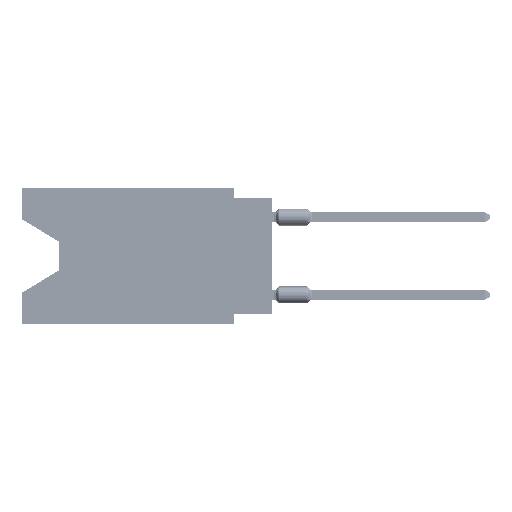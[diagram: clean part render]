
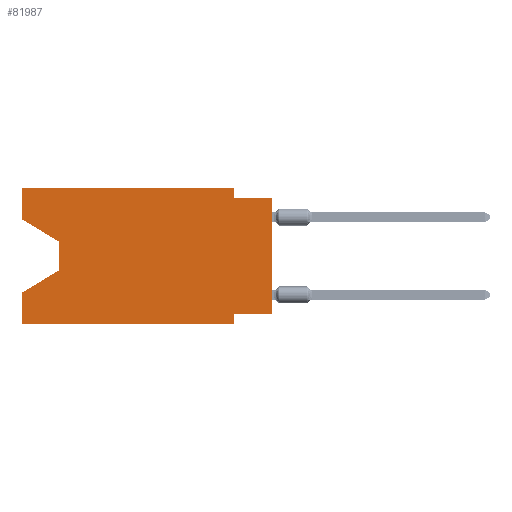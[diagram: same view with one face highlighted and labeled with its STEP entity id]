
A CAD part, left-side view. The second image highlights one B-rep face of the part: STEP entity #81987.
In plain terms, the highlighted planar face has unit normal (-1, 0, 0).
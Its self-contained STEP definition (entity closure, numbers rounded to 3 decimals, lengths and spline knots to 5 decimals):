
#1420 = ORIENTED_EDGE ( 'NONE', *, *, #66123, .F. ) ;
#2248 = CARTESIAN_POINT ( 'NONE',  ( 0., 0.1, 0. ) ) ;
#4066 = CARTESIAN_POINT ( 'NONE',  ( 0., 0., -0.025 ) ) ;
#5635 = CARTESIAN_POINT ( 'NONE',  ( 0., 0.1, 0. ) ) ;
#6984 = DIRECTION ( 'NONE',  ( 0., 0., 1. ) ) ;
#7235 = EDGE_CURVE ( 'NONE', #94374, #104248, #103990, .T. ) ;
#7316 = EDGE_CURVE ( 'NONE', #76693, #97831, #39290, .T. ) ;
#7491 = VECTOR ( 'NONE', #50959, 39.37008 ) ;
#8498 = VERTEX_POINT ( 'NONE', #97452 ) ;
#8742 = CARTESIAN_POINT ( 'NONE',  ( 0., 0.645, -0.08025 ) ) ;
#9083 = PLANE ( 'NONE',  #58738 ) ;
#9552 = ORIENTED_EDGE ( 'NONE', *, *, #91887, .T. ) ;
#11982 = EDGE_CURVE ( 'NONE', #67965, #97831, #14942, .T. ) ;
#13612 = DIRECTION ( 'NONE',  ( 0., 0.855, -0.519 ) ) ;
#14942 = LINE ( 'NONE', #64199, #66154 ) ;
#15648 = EDGE_CURVE ( 'NONE', #8498, #67965, #65523, .T. ) ;
#17375 = CARTESIAN_POINT ( 'NONE',  ( 0., 0.645, -0.35 ) ) ;
#18343 = VECTOR ( 'NONE', #51756, 39.37008 ) ;
#20702 = CARTESIAN_POINT ( 'NONE',  ( 0., 0.645, 0. ) ) ;
#21018 = VECTOR ( 'NONE', #53759, 39.37008 ) ;
#22315 = EDGE_CURVE ( 'NONE', #71827, #63925, #92590, .T. ) ;
#25149 = VECTOR ( 'NONE', #40862, 39.37008 ) ;
#27278 = CARTESIAN_POINT ( 'NONE',  ( 0., 0.645, -0.08025 ) ) ;
#28322 = VECTOR ( 'NONE', #45934, 39.37008 ) ;
#30751 = ORIENTED_EDGE ( 'NONE', *, *, #89442, .T. ) ;
#31068 = LINE ( 'NONE', #79858, #28322 ) ;
#31096 = CARTESIAN_POINT ( 'NONE',  ( 0., 0.645, -0.26975 ) ) ;
#33434 = CARTESIAN_POINT ( 'NONE',  ( 0., 0.645, 0. ) ) ;
#33614 = ORIENTED_EDGE ( 'NONE', *, *, #89465, .F. ) ;
#35167 = VECTOR ( 'NONE', #75363, 39.37008 ) ;
#35398 = EDGE_LOOP ( 'NONE', ( #9552, #64663, #30751, #1420, #56601, #73350, #79388, #45884, #54198, #80116, #33614, #39908 ) ) ;
#36526 = VERTEX_POINT ( 'NONE', #89212 ) ;
#37325 = LINE ( 'NONE', #62750, #21018 ) ;
#38444 = VECTOR ( 'NONE', #13612, 39.37008 ) ;
#39290 = LINE ( 'NONE', #39818, #25149 ) ;
#39818 = CARTESIAN_POINT ( 'NONE',  ( 0., 0.645, -0.35 ) ) ;
#39908 = ORIENTED_EDGE ( 'NONE', *, *, #7235, .F. ) ;
#40862 = DIRECTION ( 'NONE',  ( 0., -1., 0. ) ) ;
#45884 = ORIENTED_EDGE ( 'NONE', *, *, #60827, .T. ) ;
#45934 = DIRECTION ( 'NONE',  ( 0., -1., 0. ) ) ;
#50959 = DIRECTION ( 'NONE',  ( 0., 0., -1. ) ) ;
#51756 = DIRECTION ( 'NONE',  ( 0., -1., 0. ) ) ;
#52948 = CARTESIAN_POINT ( 'NONE',  ( 0., 0.1, -0.35 ) ) ;
#53759 = DIRECTION ( 'NONE',  ( 0., 0., 1. ) ) ;
#53870 = LINE ( 'NONE', #87808, #38444 ) ;
#54198 = ORIENTED_EDGE ( 'NONE', *, *, #22315, .F. ) ;
#54423 = VECTOR ( 'NONE', #6984, 39.37008 ) ;
#56601 = ORIENTED_EDGE ( 'NONE', *, *, #7316, .T. ) ;
#56765 = CARTESIAN_POINT ( 'NONE',  ( 0., 0.1, -0.325 ) ) ;
#57824 = DIRECTION ( 'NONE',  ( 1., 0., 0. ) ) ;
#58184 = DIRECTION ( 'NONE',  ( 0., 0., -1. ) ) ;
#58381 = VECTOR ( 'NONE', #66569, 39.37008 ) ;
#58738 = AXIS2_PLACEMENT_3D ( 'NONE', #33434, #57824, #65777 ) ;
#60690 = LINE ( 'NONE', #61725, #91471 ) ;
#60827 = EDGE_CURVE ( 'NONE', #8498, #63925, #60690, .T. ) ;
#61725 = CARTESIAN_POINT ( 'NONE',  ( 0., 0., 0. ) ) ;
#62750 = CARTESIAN_POINT ( 'NONE',  ( 0., 0.645, 0. ) ) ;
#63148 = CARTESIAN_POINT ( 'NONE',  ( 0., 0.645, 0. ) ) ;
#63925 = VERTEX_POINT ( 'NONE', #80502 ) ;
#64067 = EDGE_CURVE ( 'NONE', #36526, #75779, #90024, .T. ) ;
#64199 = CARTESIAN_POINT ( 'NONE',  ( 0., 0.1, -0.35 ) ) ;
#64279 = CARTESIAN_POINT ( 'NONE',  ( 0., 0.1, -0.025 ) ) ;
#64663 = ORIENTED_EDGE ( 'NONE', *, *, #64067, .T. ) ;
#65523 = LINE ( 'NONE', #80415, #58381 ) ;
#65777 = DIRECTION ( 'NONE',  ( 0., 0., -1. ) ) ;
#66123 = EDGE_CURVE ( 'NONE', #76693, #70131, #37325, .T. ) ;
#66154 = VECTOR ( 'NONE', #89672, 39.37008 ) ;
#66569 = DIRECTION ( 'NONE',  ( 0., 1., 0. ) ) ;
#67965 = VERTEX_POINT ( 'NONE', #56765 ) ;
#70131 = VERTEX_POINT ( 'NONE', #31096 ) ;
#71827 = VERTEX_POINT ( 'NONE', #64279 ) ;
#72234 = CARTESIAN_POINT ( 'NONE',  ( 0., 0.55, -0.212 ) ) ;
#73350 = ORIENTED_EDGE ( 'NONE', *, *, #11982, .F. ) ;
#75363 = DIRECTION ( 'NONE',  ( 0., -0.855, -0.519 ) ) ;
#75779 = VERTEX_POINT ( 'NONE', #72234 ) ;
#76693 = VERTEX_POINT ( 'NONE', #17375 ) ;
#77124 = DIRECTION ( 'NONE',  ( 0., 0., 1. ) ) ;
#78241 = VECTOR ( 'NONE', #58184, 39.37008 ) ;
#79388 = ORIENTED_EDGE ( 'NONE', *, *, #15648, .F. ) ;
#79858 = CARTESIAN_POINT ( 'NONE',  ( 0., 0.645, 0. ) ) ;
#80116 = ORIENTED_EDGE ( 'NONE', *, *, #100584, .F. ) ;
#80415 = CARTESIAN_POINT ( 'NONE',  ( 0., 0., -0.325 ) ) ;
#80502 = CARTESIAN_POINT ( 'NONE',  ( 0., 0., -0.025 ) ) ;
#81711 = FACE_OUTER_BOUND ( 'NONE', #35398, .T. ) ;
#81987 = ADVANCED_FACE ( 'NONE', ( #81711 ), #9083, .F. ) ;
#87808 = CARTESIAN_POINT ( 'NONE',  ( 0., 0.55, -0.212 ) ) ;
#89212 = CARTESIAN_POINT ( 'NONE',  ( 0., 0.55, -0.138 ) ) ;
#89326 = LINE ( 'NONE', #8742, #35167 ) ;
#89442 = EDGE_CURVE ( 'NONE', #75779, #70131, #53870, .T. ) ;
#89465 = EDGE_CURVE ( 'NONE', #104248, #92987, #31068, .T. ) ;
#89672 = DIRECTION ( 'NONE',  ( 0., 0., -1. ) ) ;
#90024 = LINE ( 'NONE', #96945, #78241 ) ;
#90745 = LINE ( 'NONE', #2248, #7491 ) ;
#91471 = VECTOR ( 'NONE', #77124, 39.37008 ) ;
#91887 = EDGE_CURVE ( 'NONE', #94374, #36526, #89326, .T. ) ;
#92590 = LINE ( 'NONE', #4066, #18343 ) ;
#92987 = VERTEX_POINT ( 'NONE', #5635 ) ;
#94374 = VERTEX_POINT ( 'NONE', #27278 ) ;
#96945 = CARTESIAN_POINT ( 'NONE',  ( 0., 0.55, -0.138 ) ) ;
#97452 = CARTESIAN_POINT ( 'NONE',  ( 0., 0., -0.325 ) ) ;
#97831 = VERTEX_POINT ( 'NONE', #52948 ) ;
#100584 = EDGE_CURVE ( 'NONE', #92987, #71827, #90745, .T. ) ;
#103990 = LINE ( 'NONE', #63148, #54423 ) ;
#104248 = VERTEX_POINT ( 'NONE', #20702 ) ;
